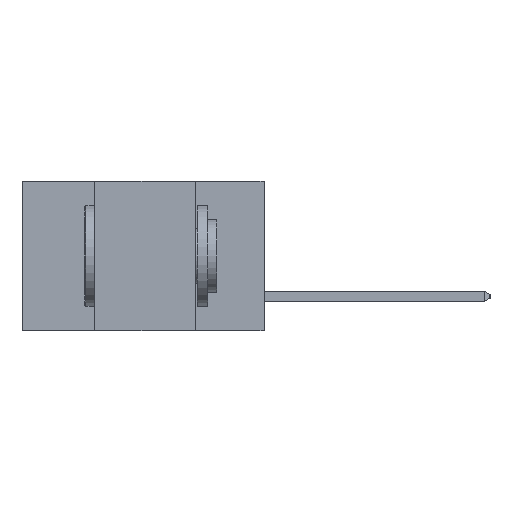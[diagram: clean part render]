
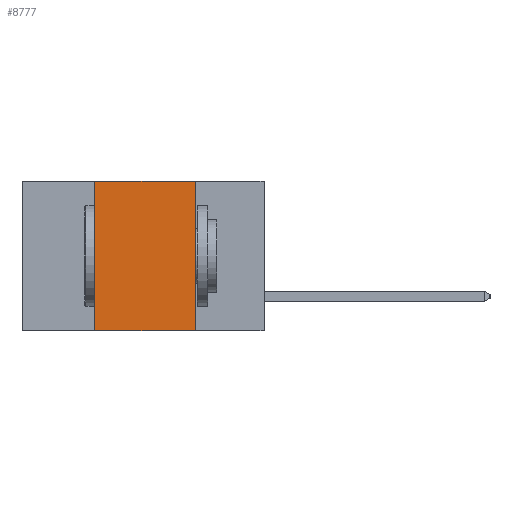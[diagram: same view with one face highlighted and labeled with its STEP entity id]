
A CAD part, left-side view. The second image highlights one B-rep face of the part: STEP entity #8777.
In plain terms, the highlighted planar face has unit normal (-1, 0, 0).
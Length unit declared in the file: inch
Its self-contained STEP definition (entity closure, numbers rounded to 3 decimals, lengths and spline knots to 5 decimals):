
#1434 = EDGE_LOOP ( 'NONE', ( #1717, #6767, #14968, #9186 ) ) ;
#1717 = ORIENTED_EDGE ( 'NONE', *, *, #9479, .F. ) ;
#2312 = CARTESIAN_POINT ( 'NONE',  ( 0., 0.17, 0. ) ) ;
#2963 = LINE ( 'NONE', #9454, #18728 ) ;
#4013 = LINE ( 'NONE', #7669, #19703 ) ;
#4014 = VERTEX_POINT ( 'NONE', #2312 ) ;
#4120 = DIRECTION ( 'NONE',  ( 0., -1., 0. ) ) ;
#4178 = CARTESIAN_POINT ( 'NONE',  ( 0., 0.6, 0. ) ) ;
#4604 = VECTOR ( 'NONE', #17382, 39.37008 ) ;
#5301 = LINE ( 'NONE', #4178, #8933 ) ;
#5332 = EDGE_CURVE ( 'NONE', #14729, #6331, #2963, .T. ) ;
#6331 = VERTEX_POINT ( 'NONE', #18285 ) ;
#6374 = EDGE_CURVE ( 'NONE', #14729, #10994, #16424, .T. ) ;
#6767 = ORIENTED_EDGE ( 'NONE', *, *, #7429, .F. ) ;
#7141 = AXIS2_PLACEMENT_3D ( 'NONE', #12567, #12389, #12383 ) ;
#7429 = EDGE_CURVE ( 'NONE', #10994, #4014, #5301, .T. ) ;
#7669 = CARTESIAN_POINT ( 'NONE',  ( 0., 0.17, -0.37 ) ) ;
#7768 = DIRECTION ( 'NONE',  ( 0., 0., -1. ) ) ;
#8777 = ADVANCED_FACE ( 'NONE', ( #17047 ), #13004, .F. ) ;
#8933 = VECTOR ( 'NONE', #4120, 39.37008 ) ;
#9186 = ORIENTED_EDGE ( 'NONE', *, *, #5332, .T. ) ;
#9454 = CARTESIAN_POINT ( 'NONE',  ( 0., 0.6, -0.37 ) ) ;
#9479 = EDGE_CURVE ( 'NONE', #4014, #6331, #4013, .T. ) ;
#9686 = DIRECTION ( 'NONE',  ( 0., -1., 0. ) ) ;
#10994 = VERTEX_POINT ( 'NONE', #17899 ) ;
#12383 = DIRECTION ( 'NONE',  ( 0., 0., -1. ) ) ;
#12389 = DIRECTION ( 'NONE',  ( 1., 0., 0. ) ) ;
#12567 = CARTESIAN_POINT ( 'NONE',  ( 0., 0.6, 0. ) ) ;
#13004 = PLANE ( 'NONE',  #7141 ) ;
#14352 = CARTESIAN_POINT ( 'NONE',  ( 0., 0.42, -0.37 ) ) ;
#14729 = VERTEX_POINT ( 'NONE', #14352 ) ;
#14968 = ORIENTED_EDGE ( 'NONE', *, *, #6374, .F. ) ;
#16424 = LINE ( 'NONE', #17367, #4604 ) ;
#17047 = FACE_OUTER_BOUND ( 'NONE', #1434, .T. ) ;
#17367 = CARTESIAN_POINT ( 'NONE',  ( 0., 0.42, -0.37 ) ) ;
#17382 = DIRECTION ( 'NONE',  ( 0., 0., 1. ) ) ;
#17899 = CARTESIAN_POINT ( 'NONE',  ( 0., 0.42, 0. ) ) ;
#18285 = CARTESIAN_POINT ( 'NONE',  ( 0., 0.17, -0.37 ) ) ;
#18728 = VECTOR ( 'NONE', #9686, 39.37008 ) ;
#19703 = VECTOR ( 'NONE', #7768, 39.37008 ) ;
